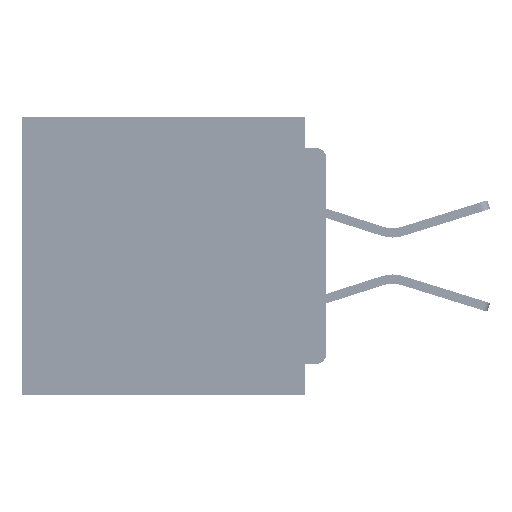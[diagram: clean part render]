
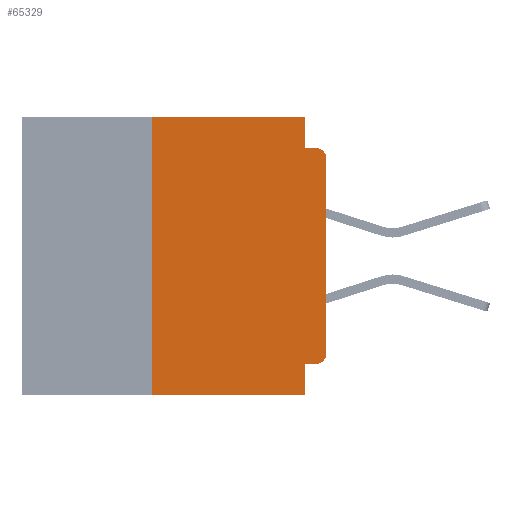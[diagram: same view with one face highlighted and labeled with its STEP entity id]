
A CAD part, left-side view. The second image highlights one B-rep face of the part: STEP entity #65329.
In plain terms, the highlighted planar face has unit normal (-1, 0, 0).
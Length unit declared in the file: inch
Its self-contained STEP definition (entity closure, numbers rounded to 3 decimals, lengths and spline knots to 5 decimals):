
#130 = LINE ( 'NONE', #21930, #27387 ) ;
#661 = ORIENTED_EDGE ( 'NONE', *, *, #67243, .F. ) ;
#894 = CARTESIAN_POINT ( 'NONE',  ( 0., 0.015, -0.34 ) ) ;
#1158 = CARTESIAN_POINT ( 'NONE',  ( 0., 0.031, -0.4 ) ) ;
#2818 = LINE ( 'NONE', #21340, #12104 ) ;
#3233 = LINE ( 'NONE', #35249, #15958 ) ;
#5448 = VERTEX_POINT ( 'NONE', #22039 ) ;
#5570 = CARTESIAN_POINT ( 'NONE',  ( 0., 0.015, -0.06 ) ) ;
#6330 = DIRECTION ( 'NONE',  ( 0., 0., -1. ) ) ;
#6494 = CARTESIAN_POINT ( 'NONE',  ( 0., 0.437, 0. ) ) ;
#10208 = CARTESIAN_POINT ( 'NONE',  ( 0., 0.437, 0. ) ) ;
#10685 = CARTESIAN_POINT ( 'NONE',  ( 0., 0.015, -0.045 ) ) ;
#10951 = EDGE_CURVE ( 'NONE', #13194, #11667, #70261, .T. ) ;
#11006 = DIRECTION ( 'NONE',  ( 0., 0., -1. ) ) ;
#11121 = EDGE_CURVE ( 'NONE', #58997, #15435, #32883, .T. ) ;
#11667 = VERTEX_POINT ( 'NONE', #1158 ) ;
#12104 = VECTOR ( 'NONE', #64910, 39.37008 ) ;
#13194 = VERTEX_POINT ( 'NONE', #61591 ) ;
#13560 = CARTESIAN_POINT ( 'NONE',  ( 0., 0., -0.355 ) ) ;
#13759 = EDGE_LOOP ( 'NONE', ( #16526, #68274, #38084, #14302, #69766, #37448, #65106, #661, #21194, #21024 ) ) ;
#14302 = ORIENTED_EDGE ( 'NONE', *, *, #42534, .F. ) ;
#14605 = CARTESIAN_POINT ( 'NONE',  ( 0., 0.25, 0. ) ) ;
#14867 = VECTOR ( 'NONE', #49326, 39.37008 ) ;
#15435 = VERTEX_POINT ( 'NONE', #60128 ) ;
#15958 = VECTOR ( 'NONE', #40712, 39.37008 ) ;
#16526 = ORIENTED_EDGE ( 'NONE', *, *, #61336, .T. ) ;
#17246 = VECTOR ( 'NONE', #37505, 39.37008 ) ;
#17597 = CARTESIAN_POINT ( 'NONE',  ( 0., 0.437, -0.4 ) ) ;
#20128 = AXIS2_PLACEMENT_3D ( 'NONE', #894, #39058, #6330 ) ;
#21024 = ORIENTED_EDGE ( 'NONE', *, *, #30857, .T. ) ;
#21194 = ORIENTED_EDGE ( 'NONE', *, *, #11121, .F. ) ;
#21340 = CARTESIAN_POINT ( 'NONE',  ( 0., 0.031, 0. ) ) ;
#21529 = CARTESIAN_POINT ( 'NONE',  ( 0., 0.015, -0.355 ) ) ;
#21930 = CARTESIAN_POINT ( 'NONE',  ( 0., 0.25, -0.4 ) ) ;
#22039 = CARTESIAN_POINT ( 'NONE',  ( 0., 0.031, 0. ) ) ;
#23872 = EDGE_CURVE ( 'NONE', #60601, #63108, #38455, .T. ) ;
#25239 = VERTEX_POINT ( 'NONE', #35017 ) ;
#26914 = VECTOR ( 'NONE', #55983, 39.37008 ) ;
#27387 = VECTOR ( 'NONE', #27460, 39.37008 ) ;
#27460 = DIRECTION ( 'NONE',  ( 0., 0., 1. ) ) ;
#29233 = VERTEX_POINT ( 'NONE', #14605 ) ;
#30177 = CARTESIAN_POINT ( 'NONE',  ( 0., 0., -0.06 ) ) ;
#30660 = VERTEX_POINT ( 'NONE', #63465 ) ;
#30857 = EDGE_CURVE ( 'NONE', #58997, #30660, #65602, .T. ) ;
#32211 = DIRECTION ( 'NONE',  ( 1., 0., 0. ) ) ;
#32883 = LINE ( 'NONE', #13560, #34587 ) ;
#34587 = VECTOR ( 'NONE', #46003, 39.37008 ) ;
#35017 = CARTESIAN_POINT ( 'NONE',  ( 0., 0.031, -0.045 ) ) ;
#35249 = CARTESIAN_POINT ( 'NONE',  ( 0., 0., -0.045 ) ) ;
#37448 = ORIENTED_EDGE ( 'NONE', *, *, #40053, .F. ) ;
#37505 = DIRECTION ( 'NONE',  ( 0., 0., 1. ) ) ;
#38084 = ORIENTED_EDGE ( 'NONE', *, *, #58669, .F. ) ;
#38455 = CIRCLE ( 'NONE', #63631, 0.015 ) ;
#39058 = DIRECTION ( 'NONE',  ( -1., 0., 0. ) ) ;
#40053 = EDGE_CURVE ( 'NONE', #13194, #29233, #130, .T. ) ;
#40229 = LINE ( 'NONE', #6494, #69075 ) ;
#40712 = DIRECTION ( 'NONE',  ( 0., -1., 0. ) ) ;
#42534 = EDGE_CURVE ( 'NONE', #5448, #25239, #2818, .T. ) ;
#43716 = DIRECTION ( 'NONE',  ( -1., 0., 0. ) ) ;
#43886 = CARTESIAN_POINT ( 'NONE',  ( 0., 0.031, -0.4 ) ) ;
#44667 = DIRECTION ( 'NONE',  ( 0., -1., 0. ) ) ;
#46003 = DIRECTION ( 'NONE',  ( 0., 1., 0. ) ) ;
#48383 = PLANE ( 'NONE',  #54372 ) ;
#48631 = EDGE_CURVE ( 'NONE', #29233, #5448, #40229, .T. ) ;
#49326 = DIRECTION ( 'NONE',  ( 0., 0., -1. ) ) ;
#54372 = AXIS2_PLACEMENT_3D ( 'NONE', #10208, #32211, #70175 ) ;
#55983 = DIRECTION ( 'NONE',  ( 0., -1., 0. ) ) ;
#58329 = LINE ( 'NONE', #43886, #14867 ) ;
#58669 = EDGE_CURVE ( 'NONE', #25239, #63108, #3233, .T. ) ;
#58997 = VERTEX_POINT ( 'NONE', #21529 ) ;
#59032 = LINE ( 'NONE', #64540, #17246 ) ;
#60128 = CARTESIAN_POINT ( 'NONE',  ( 0., 0.031, -0.355 ) ) ;
#60601 = VERTEX_POINT ( 'NONE', #30177 ) ;
#61336 = EDGE_CURVE ( 'NONE', #30660, #60601, #59032, .T. ) ;
#61591 = CARTESIAN_POINT ( 'NONE',  ( 0., 0.25, -0.4 ) ) ;
#63108 = VERTEX_POINT ( 'NONE', #10685 ) ;
#63465 = CARTESIAN_POINT ( 'NONE',  ( 0., 0., -0.34 ) ) ;
#63631 = AXIS2_PLACEMENT_3D ( 'NONE', #5570, #43716, #11006 ) ;
#64540 = CARTESIAN_POINT ( 'NONE',  ( 0., 0., 0. ) ) ;
#64910 = DIRECTION ( 'NONE',  ( 0., 0., -1. ) ) ;
#65106 = ORIENTED_EDGE ( 'NONE', *, *, #10951, .T. ) ;
#65329 = ADVANCED_FACE ( 'NONE', ( #68792 ), #48383, .F. ) ;
#65602 = CIRCLE ( 'NONE', #20128, 0.015 ) ;
#67243 = EDGE_CURVE ( 'NONE', #15435, #11667, #58329, .T. ) ;
#68274 = ORIENTED_EDGE ( 'NONE', *, *, #23872, .T. ) ;
#68792 = FACE_OUTER_BOUND ( 'NONE', #13759, .T. ) ;
#69075 = VECTOR ( 'NONE', #44667, 39.37008 ) ;
#69766 = ORIENTED_EDGE ( 'NONE', *, *, #48631, .F. ) ;
#70175 = DIRECTION ( 'NONE',  ( 0., 0., -1. ) ) ;
#70261 = LINE ( 'NONE', #17597, #26914 ) ;
